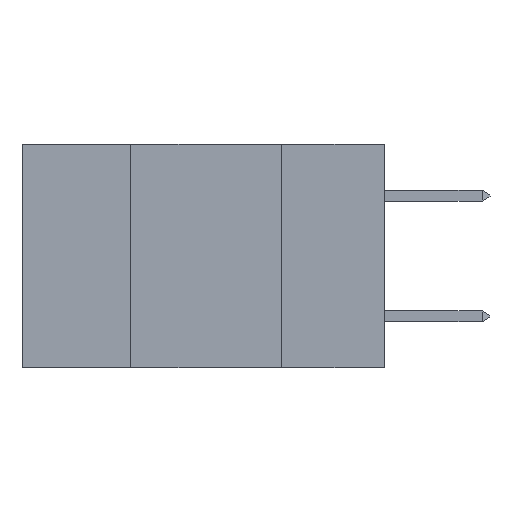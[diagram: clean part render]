
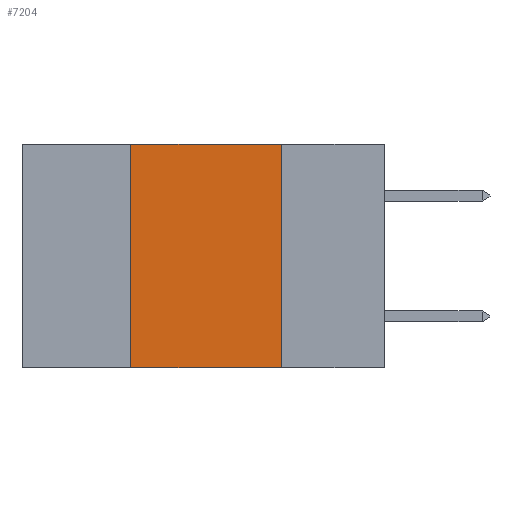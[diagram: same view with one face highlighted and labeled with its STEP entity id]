
A CAD part, left-side view. The second image highlights one B-rep face of the part: STEP entity #7204.
In plain terms, the highlighted planar face has unit normal (-1, 0, 0).
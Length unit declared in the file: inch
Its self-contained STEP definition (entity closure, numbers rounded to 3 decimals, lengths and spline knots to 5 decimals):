
#366 = EDGE_CURVE ( 'NONE', #809, #8477, #11671, .T. ) ;
#421 = CARTESIAN_POINT ( 'NONE',  ( 0., 0.6, 0. ) ) ;
#809 = VERTEX_POINT ( 'NONE', #5518 ) ;
#1567 = EDGE_CURVE ( 'NONE', #3037, #809, #11885, .T. ) ;
#2024 = CARTESIAN_POINT ( 'NONE',  ( 0., 0.6, -0.37 ) ) ;
#2287 = CARTESIAN_POINT ( 'NONE',  ( 0., 0.42, 0. ) ) ;
#2606 = CARTESIAN_POINT ( 'NONE',  ( 0., 0.17, 0. ) ) ;
#2643 = VECTOR ( 'NONE', #6436, 39.37008 ) ;
#2770 = VERTEX_POINT ( 'NONE', #12241 ) ;
#3037 = VERTEX_POINT ( 'NONE', #12274 ) ;
#3108 = DIRECTION ( 'NONE',  ( 0., -1., 0. ) ) ;
#4492 = ORIENTED_EDGE ( 'NONE', *, *, #8273, .T. ) ;
#4760 = DIRECTION ( 'NONE',  ( 0., 0., -1. ) ) ;
#5518 = CARTESIAN_POINT ( 'NONE',  ( 0., 0.17, 0. ) ) ;
#5543 = DIRECTION ( 'NONE',  ( 0., -1., 0. ) ) ;
#6169 = VECTOR ( 'NONE', #3108, 39.37008 ) ;
#6436 = DIRECTION ( 'NONE',  ( 0., 0., 1. ) ) ;
#6476 = DIRECTION ( 'NONE',  ( 0., 0., -1. ) ) ;
#6647 = CARTESIAN_POINT ( 'NONE',  ( 0., 0.6, 0. ) ) ;
#7204 = ADVANCED_FACE ( 'NONE', ( #13004 ), #9865, .F. ) ;
#7577 = ORIENTED_EDGE ( 'NONE', *, *, #1567, .F. ) ;
#7798 = DIRECTION ( 'NONE',  ( 1., 0., 0. ) ) ;
#8273 = EDGE_CURVE ( 'NONE', #2770, #8477, #9257, .T. ) ;
#8477 = VERTEX_POINT ( 'NONE', #10477 ) ;
#8930 = ORIENTED_EDGE ( 'NONE', *, *, #9048, .F. ) ;
#9048 = EDGE_CURVE ( 'NONE', #2770, #3037, #11624, .T. ) ;
#9257 = LINE ( 'NONE', #2024, #6169 ) ;
#9360 = AXIS2_PLACEMENT_3D ( 'NONE', #6647, #7798, #4760 ) ;
#9865 = PLANE ( 'NONE',  #9360 ) ;
#9923 = EDGE_LOOP ( 'NONE', ( #11899, #7577, #8930, #4492 ) ) ;
#10072 = VECTOR ( 'NONE', #5543, 39.37008 ) ;
#10411 = VECTOR ( 'NONE', #6476, 39.37008 ) ;
#10477 = CARTESIAN_POINT ( 'NONE',  ( 0., 0.17, -0.37 ) ) ;
#11624 = LINE ( 'NONE', #2287, #2643 ) ;
#11671 = LINE ( 'NONE', #2606, #10411 ) ;
#11885 = LINE ( 'NONE', #421, #10072 ) ;
#11899 = ORIENTED_EDGE ( 'NONE', *, *, #366, .F. ) ;
#12241 = CARTESIAN_POINT ( 'NONE',  ( 0., 0.42, -0.37 ) ) ;
#12274 = CARTESIAN_POINT ( 'NONE',  ( 0., 0.42, 0. ) ) ;
#13004 = FACE_OUTER_BOUND ( 'NONE', #9923, .T. ) ;
